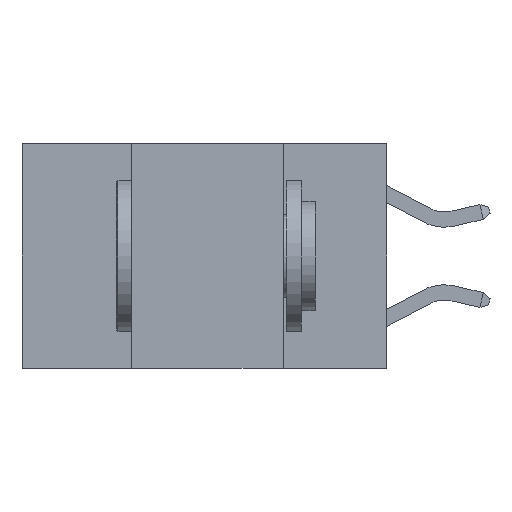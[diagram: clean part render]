
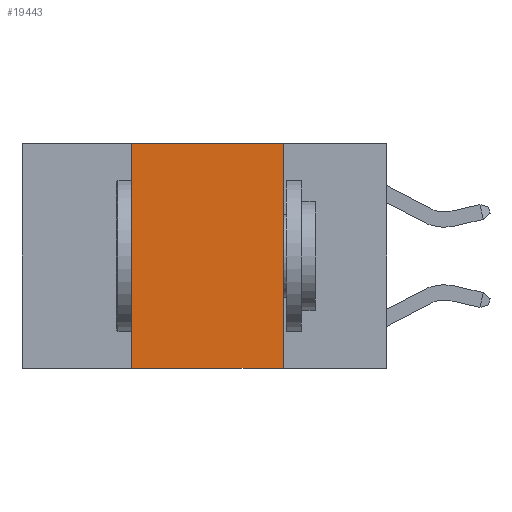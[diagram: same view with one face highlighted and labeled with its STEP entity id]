
A CAD part, left-side view. The second image highlights one B-rep face of the part: STEP entity #19443.
In plain terms, the highlighted planar face has unit normal (-1, 0, 0).
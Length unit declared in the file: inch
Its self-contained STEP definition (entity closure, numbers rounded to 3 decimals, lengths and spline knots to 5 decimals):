
#817 = FACE_OUTER_BOUND ( 'NONE', #21475, .T. ) ;
#1062 = DIRECTION ( 'NONE',  ( 0., 0., -1. ) ) ;
#1670 = DIRECTION ( 'NONE',  ( 0., 0., -1. ) ) ;
#3045 = VERTEX_POINT ( 'NONE', #5690 ) ;
#3162 = VERTEX_POINT ( 'NONE', #28536 ) ;
#3340 = CARTESIAN_POINT ( 'NONE',  ( 0., 0.17, 0. ) ) ;
#4320 = VECTOR ( 'NONE', #7938, 39.37008 ) ;
#4437 = ORIENTED_EDGE ( 'NONE', *, *, #7235, .F. ) ;
#4836 = VECTOR ( 'NONE', #23985, 39.37008 ) ;
#5528 = LINE ( 'NONE', #22322, #4836 ) ;
#5690 = CARTESIAN_POINT ( 'NONE',  ( 0., 0.17, -0.37 ) ) ;
#7235 = EDGE_CURVE ( 'NONE', #3162, #12706, #5528, .T. ) ;
#7640 = LINE ( 'NONE', #8084, #4320 ) ;
#7938 = DIRECTION ( 'NONE',  ( 0., -1., 0. ) ) ;
#8084 = CARTESIAN_POINT ( 'NONE',  ( 0., 0.6, -0.37 ) ) ;
#8488 = ORIENTED_EDGE ( 'NONE', *, *, #13896, .F. ) ;
#9253 = AXIS2_PLACEMENT_3D ( 'NONE', #17045, #10198, #1670 ) ;
#10198 = DIRECTION ( 'NONE',  ( 1., 0., 0. ) ) ;
#12261 = CARTESIAN_POINT ( 'NONE',  ( 0., 0.42, -0.37 ) ) ;
#12706 = VERTEX_POINT ( 'NONE', #3340 ) ;
#12733 = EDGE_CURVE ( 'NONE', #12706, #3045, #24221, .T. ) ;
#13896 = EDGE_CURVE ( 'NONE', #22024, #3162, #19395, .T. ) ;
#14890 = VECTOR ( 'NONE', #28615, 39.37008 ) ;
#15268 = EDGE_CURVE ( 'NONE', #22024, #3045, #7640, .T. ) ;
#17045 = CARTESIAN_POINT ( 'NONE',  ( 0., 0.6, 0. ) ) ;
#17588 = PLANE ( 'NONE',  #9253 ) ;
#19395 = LINE ( 'NONE', #23936, #14890 ) ;
#19443 = ADVANCED_FACE ( 'NONE', ( #817 ), #17588, .F. ) ;
#21475 = EDGE_LOOP ( 'NONE', ( #26089, #4437, #8488, #22882 ) ) ;
#22024 = VERTEX_POINT ( 'NONE', #12261 ) ;
#22322 = CARTESIAN_POINT ( 'NONE',  ( 0., 0.6, 0. ) ) ;
#22882 = ORIENTED_EDGE ( 'NONE', *, *, #15268, .T. ) ;
#23936 = CARTESIAN_POINT ( 'NONE',  ( 0., 0.42, 0. ) ) ;
#23985 = DIRECTION ( 'NONE',  ( 0., -1., 0. ) ) ;
#24221 = LINE ( 'NONE', #28606, #26444 ) ;
#26089 = ORIENTED_EDGE ( 'NONE', *, *, #12733, .F. ) ;
#26444 = VECTOR ( 'NONE', #1062, 39.37008 ) ;
#28536 = CARTESIAN_POINT ( 'NONE',  ( 0., 0.42, 0. ) ) ;
#28606 = CARTESIAN_POINT ( 'NONE',  ( 0., 0.17, 0. ) ) ;
#28615 = DIRECTION ( 'NONE',  ( 0., 0., 1. ) ) ;
